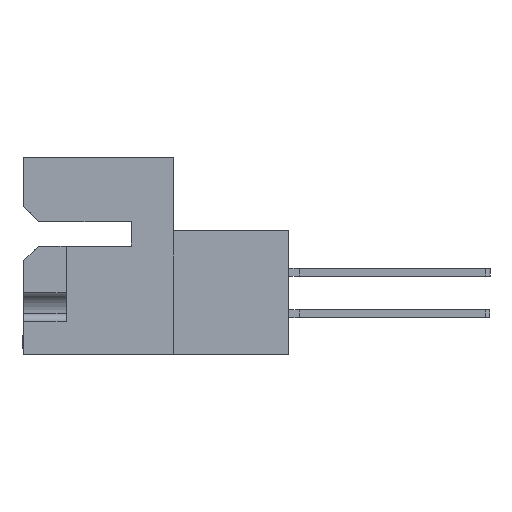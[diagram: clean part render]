
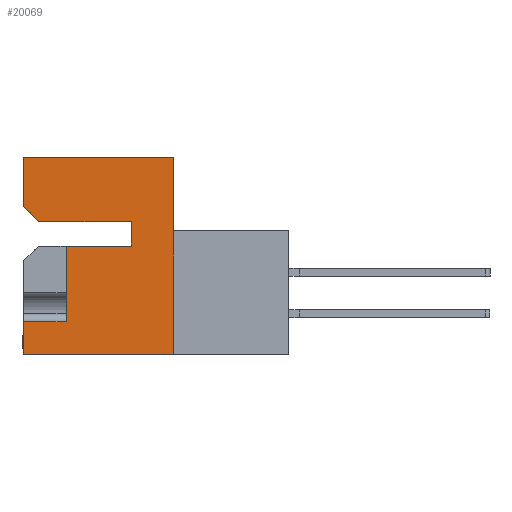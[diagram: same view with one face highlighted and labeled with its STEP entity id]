
A CAD part, left-side view. The second image highlights one B-rep face of the part: STEP entity #20069.
In plain terms, the highlighted planar face has unit normal (-1, 0, 0).
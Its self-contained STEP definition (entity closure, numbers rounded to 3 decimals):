
#3038 = AXIS2_PLACEMENT_3D ( 'NONE', #47360, #23472, #35640 ) ;
#5345 = EDGE_CURVE ( 'NONE', #21798, #12268, #40679, .T. ) ;
#5607 = VERTEX_POINT ( 'NONE', #45925 ) ;
#6348 = VECTOR ( 'NONE', #20242, 1000. ) ;
#6616 = VERTEX_POINT ( 'NONE', #37757 ) ;
#6663 = CARTESIAN_POINT ( 'NONE',  ( 0., 3.251, -6.782 ) ) ;
#7533 = DIRECTION ( 'NONE',  ( 0., 1., 0. ) ) ;
#10326 = VECTOR ( 'NONE', #24338, 1000. ) ;
#11435 = ORIENTED_EDGE ( 'NONE', *, *, #33328, .F. ) ;
#12048 = FACE_OUTER_BOUND ( 'NONE', #46517, .T. ) ;
#12123 = VERTEX_POINT ( 'NONE', #39778 ) ;
#12268 = VERTEX_POINT ( 'NONE', #29122 ) ;
#12512 = EDGE_CURVE ( 'NONE', #45937, #24614, #15579, .T. ) ;
#12901 = VECTOR ( 'NONE', #39294, 1000. ) ;
#12923 = EDGE_CURVE ( 'NONE', #37321, #12268, #34453, .T. ) ;
#14064 = CARTESIAN_POINT ( 'NONE',  ( 0., 0., 0. ) ) ;
#14070 = VECTOR ( 'NONE', #51243, 1000. ) ;
#14758 = EDGE_CURVE ( 'NONE', #6616, #24614, #30571, .T. ) ;
#14853 = EDGE_CURVE ( 'NONE', #25609, #12123, #29334, .T. ) ;
#15004 = DIRECTION ( 'NONE',  ( 0., 0., 1. ) ) ;
#15182 = LINE ( 'NONE', #14064, #40800 ) ;
#15579 = LINE ( 'NONE', #35786, #33056 ) ;
#16030 = LINE ( 'NONE', #31089, #12901 ) ;
#16382 = VECTOR ( 'NONE', #45493, 1000. ) ;
#17226 = ORIENTED_EDGE ( 'NONE', *, *, #5345, .T. ) ;
#18237 = ORIENTED_EDGE ( 'NONE', *, *, #12512, .T. ) ;
#19493 = ORIENTED_EDGE ( 'NONE', *, *, #14853, .F. ) ;
#19611 = DIRECTION ( 'NONE',  ( 0., -0.707, -0.707 ) ) ;
#19979 = VECTOR ( 'NONE', #7533, 1000. ) ;
#20069 = ADVANCED_FACE ( 'NONE', ( #12048 ), #43365, .F. ) ;
#20242 = DIRECTION ( 'NONE',  ( 0., 0., 1. ) ) ;
#21758 = CARTESIAN_POINT ( 'NONE',  ( 0., 0., -15.088 ) ) ;
#21798 = VERTEX_POINT ( 'NONE', #48796 ) ;
#21978 = LINE ( 'NONE', #44812, #6348 ) ;
#22191 = VECTOR ( 'NONE', #15004, 1000. ) ;
#23370 = EDGE_CURVE ( 'NONE', #45937, #23762, #21978, .T. ) ;
#23472 = DIRECTION ( 'NONE',  ( 1., 0., 0. ) ) ;
#23762 = VERTEX_POINT ( 'NONE', #51789 ) ;
#24102 = ORIENTED_EDGE ( 'NONE', *, *, #12923, .F. ) ;
#24338 = DIRECTION ( 'NONE',  ( 0., 1., 0. ) ) ;
#24614 = VERTEX_POINT ( 'NONE', #49097 ) ;
#25609 = VERTEX_POINT ( 'NONE', #34218 ) ;
#28482 = CARTESIAN_POINT ( 'NONE',  ( 0., 8.255, -12.58 ) ) ;
#28684 = VECTOR ( 'NONE', #32623, 1000. ) ;
#29122 = CARTESIAN_POINT ( 'NONE',  ( 0., 11.506, -12.58 ) ) ;
#29334 = LINE ( 'NONE', #32105, #28684 ) ;
#30571 = LINE ( 'NONE', #47312, #19979 ) ;
#30819 = CARTESIAN_POINT ( 'NONE',  ( 0., 8.255, -6.782 ) ) ;
#30890 = ORIENTED_EDGE ( 'NONE', *, *, #14758, .F. ) ;
#31089 = CARTESIAN_POINT ( 'NONE',  ( 0., 11.506, 0. ) ) ;
#31623 = DIRECTION ( 'NONE',  ( 0., 1., 0. ) ) ;
#31651 = CARTESIAN_POINT ( 'NONE',  ( 0., -8.814, -15.088 ) ) ;
#32105 = CARTESIAN_POINT ( 'NONE',  ( 0., 0., -6.782 ) ) ;
#32623 = DIRECTION ( 'NONE',  ( 0., -1., 0. ) ) ;
#33056 = VECTOR ( 'NONE', #19611, 1000. ) ;
#33328 = EDGE_CURVE ( 'NONE', #47508, #37321, #38419, .T. ) ;
#33700 = EDGE_CURVE ( 'NONE', #12123, #6616, #43398, .T. ) ;
#34030 = ORIENTED_EDGE ( 'NONE', *, *, #37621, .F. ) ;
#34218 = CARTESIAN_POINT ( 'NONE',  ( 0., 8.255, -6.782 ) ) ;
#34453 = LINE ( 'NONE', #37780, #16382 ) ;
#35640 = DIRECTION ( 'NONE',  ( 0., 0., -1. ) ) ;
#35786 = CARTESIAN_POINT ( 'NONE',  ( 0., 10.363, -4.902 ) ) ;
#35821 = CARTESIAN_POINT ( 'NONE',  ( 0., 11.506, -15.088 ) ) ;
#37321 = VERTEX_POINT ( 'NONE', #35821 ) ;
#37364 = ORIENTED_EDGE ( 'NONE', *, *, #33700, .F. ) ;
#37621 = EDGE_CURVE ( 'NONE', #5607, #47508, #15182, .T. ) ;
#37757 = CARTESIAN_POINT ( 'NONE',  ( 0., 3.251, -4.902 ) ) ;
#37780 = CARTESIAN_POINT ( 'NONE',  ( 0., 11.506, -15.088 ) ) ;
#37816 = DIRECTION ( 'NONE',  ( 0., 0., -1. ) ) ;
#38050 = ORIENTED_EDGE ( 'NONE', *, *, #42581, .F. ) ;
#38419 = LINE ( 'NONE', #31651, #10326 ) ;
#39294 = DIRECTION ( 'NONE',  ( 0., -1., 0. ) ) ;
#39778 = CARTESIAN_POINT ( 'NONE',  ( 0., 3.251, -6.782 ) ) ;
#40582 = VECTOR ( 'NONE', #31623, 1000. ) ;
#40679 = LINE ( 'NONE', #28482, #40582 ) ;
#40800 = VECTOR ( 'NONE', #37816, 1000. ) ;
#42581 = EDGE_CURVE ( 'NONE', #23762, #5607, #16030, .T. ) ;
#43047 = ORIENTED_EDGE ( 'NONE', *, *, #43399, .F. ) ;
#43365 = PLANE ( 'NONE',  #3038 ) ;
#43398 = LINE ( 'NONE', #6663, #22191 ) ;
#43399 = EDGE_CURVE ( 'NONE', #21798, #25609, #45363, .T. ) ;
#44812 = CARTESIAN_POINT ( 'NONE',  ( 0., 11.506, -15.088 ) ) ;
#45363 = LINE ( 'NONE', #30819, #14070 ) ;
#45493 = DIRECTION ( 'NONE',  ( 0., 0., 1. ) ) ;
#45925 = CARTESIAN_POINT ( 'NONE',  ( 0., 0., 0. ) ) ;
#45937 = VERTEX_POINT ( 'NONE', #46010 ) ;
#46010 = CARTESIAN_POINT ( 'NONE',  ( 0., 11.506, -3.759 ) ) ;
#46517 = EDGE_LOOP ( 'NONE', ( #11435, #34030, #38050, #47384, #18237, #30890, #37364, #19493, #43047, #17226, #24102 ) ) ;
#47312 = CARTESIAN_POINT ( 'NONE',  ( 0., 0., -4.902 ) ) ;
#47360 = CARTESIAN_POINT ( 'NONE',  ( 0., 0., 0. ) ) ;
#47384 = ORIENTED_EDGE ( 'NONE', *, *, #23370, .F. ) ;
#47508 = VERTEX_POINT ( 'NONE', #21758 ) ;
#48796 = CARTESIAN_POINT ( 'NONE',  ( 0., 8.255, -12.58 ) ) ;
#49097 = CARTESIAN_POINT ( 'NONE',  ( 0., 10.363, -4.902 ) ) ;
#51243 = DIRECTION ( 'NONE',  ( 0., 0., 1. ) ) ;
#51789 = CARTESIAN_POINT ( 'NONE',  ( 0., 11.506, 0. ) ) ;
